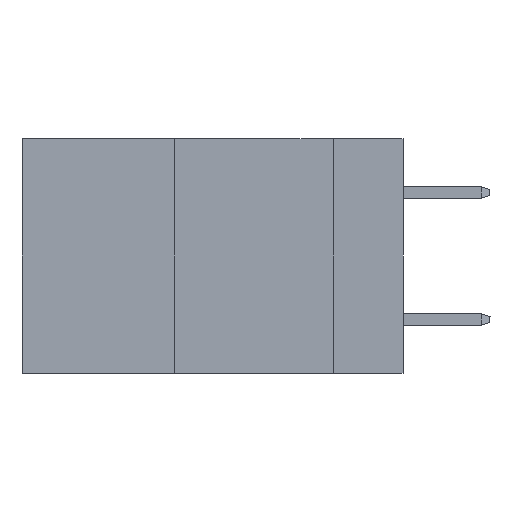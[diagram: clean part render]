
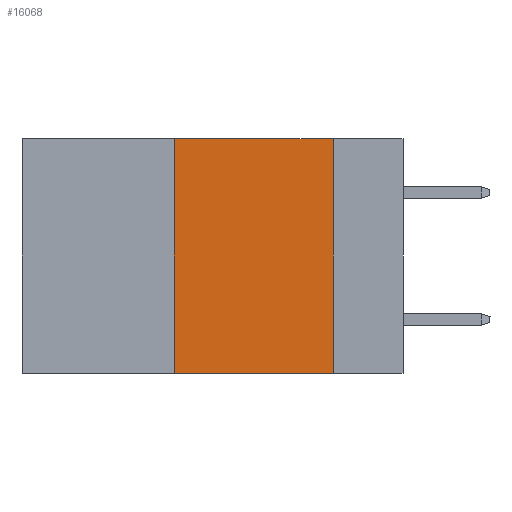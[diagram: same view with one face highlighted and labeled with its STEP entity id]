
A CAD part, left-side view. The second image highlights one B-rep face of the part: STEP entity #16068.
In plain terms, the highlighted planar face has unit normal (-1, 0, 0).
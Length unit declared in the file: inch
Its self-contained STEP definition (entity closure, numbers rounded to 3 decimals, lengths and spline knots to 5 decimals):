
#1642 = PLANE ( 'NONE',  #15463 ) ;
#1778 = VECTOR ( 'NONE', #2920, 39.37008 ) ;
#2920 = DIRECTION ( 'NONE',  ( 0., 0., -1. ) ) ;
#4353 = ORIENTED_EDGE ( 'NONE', *, *, #9442, .F. ) ;
#5286 = DIRECTION ( 'NONE',  ( 0., -1., 0. ) ) ;
#5483 = CARTESIAN_POINT ( 'NONE',  ( 0., 0.11, 0. ) ) ;
#5635 = CARTESIAN_POINT ( 'NONE',  ( 0., 0.6, 0. ) ) ;
#6224 = DIRECTION ( 'NONE',  ( 1., 0., 0. ) ) ;
#6469 = VERTEX_POINT ( 'NONE', #16195 ) ;
#6584 = EDGE_LOOP ( 'NONE', ( #7817, #25108, #4353, #8487 ) ) ;
#7817 = ORIENTED_EDGE ( 'NONE', *, *, #19267, .F. ) ;
#8140 = VECTOR ( 'NONE', #5286, 39.37008 ) ;
#8453 = FACE_OUTER_BOUND ( 'NONE', #6584, .T. ) ;
#8487 = ORIENTED_EDGE ( 'NONE', *, *, #9047, .T. ) ;
#9047 = EDGE_CURVE ( 'NONE', #27389, #18932, #23273, .T. ) ;
#9442 = EDGE_CURVE ( 'NONE', #27389, #6469, #23238, .T. ) ;
#9917 = LINE ( 'NONE', #12188, #1778 ) ;
#12188 = CARTESIAN_POINT ( 'NONE',  ( 0., 0.11, 0. ) ) ;
#14182 = EDGE_CURVE ( 'NONE', #6469, #24906, #18502, .T. ) ;
#14199 = DIRECTION ( 'NONE',  ( 0., -1., 0. ) ) ;
#14349 = CARTESIAN_POINT ( 'NONE',  ( 0., 0.6, 0. ) ) ;
#14403 = CARTESIAN_POINT ( 'NONE',  ( 0., 0.6, -0.37 ) ) ;
#15350 = CARTESIAN_POINT ( 'NONE',  ( 0., 0.11, -0.37 ) ) ;
#15457 = VECTOR ( 'NONE', #14199, 39.37008 ) ;
#15463 = AXIS2_PLACEMENT_3D ( 'NONE', #5635, #6224, #22021 ) ;
#16068 = ADVANCED_FACE ( 'NONE', ( #8453 ), #1642, .F. ) ;
#16195 = CARTESIAN_POINT ( 'NONE',  ( 0., 0.36, 0. ) ) ;
#18372 = DIRECTION ( 'NONE',  ( 0., 0., 1. ) ) ;
#18502 = LINE ( 'NONE', #14349, #15457 ) ;
#18932 = VERTEX_POINT ( 'NONE', #15350 ) ;
#19267 = EDGE_CURVE ( 'NONE', #24906, #18932, #9917, .T. ) ;
#20750 = CARTESIAN_POINT ( 'NONE',  ( 0., 0.36, 0. ) ) ;
#21928 = VECTOR ( 'NONE', #18372, 39.37008 ) ;
#22021 = DIRECTION ( 'NONE',  ( 0., 0., -1. ) ) ;
#23238 = LINE ( 'NONE', #20750, #21928 ) ;
#23273 = LINE ( 'NONE', #14403, #8140 ) ;
#23878 = CARTESIAN_POINT ( 'NONE',  ( 0., 0.36, -0.37 ) ) ;
#24906 = VERTEX_POINT ( 'NONE', #5483 ) ;
#25108 = ORIENTED_EDGE ( 'NONE', *, *, #14182, .F. ) ;
#27389 = VERTEX_POINT ( 'NONE', #23878 ) ;
